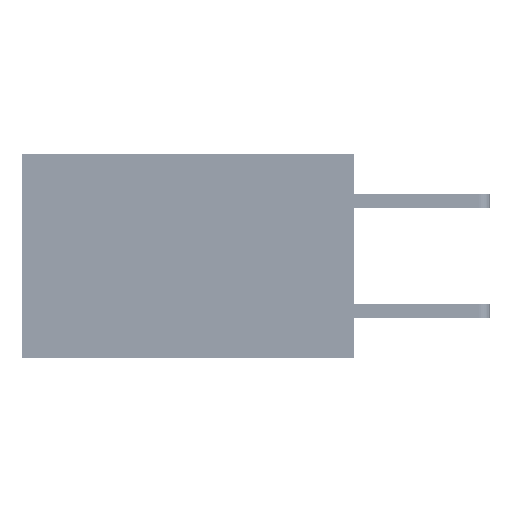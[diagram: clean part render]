
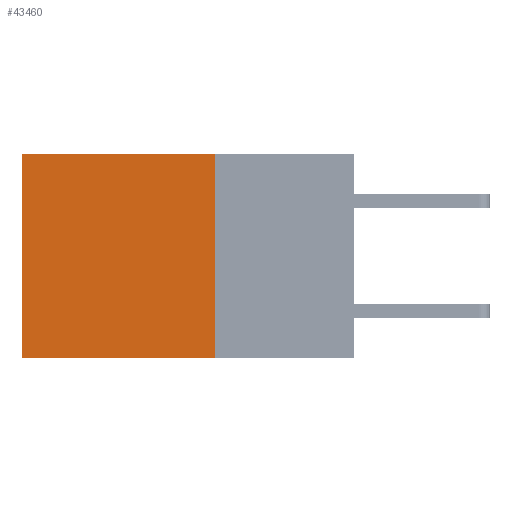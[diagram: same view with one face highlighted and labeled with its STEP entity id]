
A CAD part, left-side view. The second image highlights one B-rep face of the part: STEP entity #43460.
In plain terms, the highlighted planar face has unit normal (-1, 0, 0).
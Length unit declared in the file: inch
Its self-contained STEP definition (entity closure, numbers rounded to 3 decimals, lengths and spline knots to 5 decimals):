
#85 = CARTESIAN_POINT ( 'NONE',  ( 0.2875, 0.25, -0.37 ) ) ;
#1577 = EDGE_CURVE ( 'NONE', #25492, #35846, #40350, .T. ) ;
#1589 = ORIENTED_EDGE ( 'NONE', *, *, #36701, .F. ) ;
#4598 = ORIENTED_EDGE ( 'NONE', *, *, #1577, .T. ) ;
#4735 = CARTESIAN_POINT ( 'NONE',  ( 0.2875, 0.6, 0. ) ) ;
#4952 = VECTOR ( 'NONE', #6982, 39.37008 ) ;
#6982 = DIRECTION ( 'NONE',  ( 0., 1., 0. ) ) ;
#8713 = CARTESIAN_POINT ( 'NONE',  ( 0.2875, 0.25, 0. ) ) ;
#10041 = FACE_OUTER_BOUND ( 'NONE', #24986, .T. ) ;
#13218 = DIRECTION ( 'NONE',  ( 0., 0., -1. ) ) ;
#15176 = VERTEX_POINT ( 'NONE', #21913 ) ;
#15737 = DIRECTION ( 'NONE',  ( 0., 0., -1. ) ) ;
#17518 = CARTESIAN_POINT ( 'NONE',  ( 0.2875, 0.25, 0. ) ) ;
#18536 = EDGE_CURVE ( 'NONE', #28150, #25492, #32830, .T. ) ;
#19465 = ORIENTED_EDGE ( 'NONE', *, *, #37865, .F. ) ;
#20955 = DIRECTION ( 'NONE',  ( 0., 1., 0. ) ) ;
#21913 = CARTESIAN_POINT ( 'NONE',  ( 0.2875, 0.25, -0.37 ) ) ;
#23087 = VECTOR ( 'NONE', #20955, 39.37008 ) ;
#24986 = EDGE_LOOP ( 'NONE', ( #4598, #1589, #19465, #33748 ) ) ;
#25492 = VERTEX_POINT ( 'NONE', #4735 ) ;
#28150 = VERTEX_POINT ( 'NONE', #37398 ) ;
#30674 = VECTOR ( 'NONE', #13218, 39.37008 ) ;
#31085 = VECTOR ( 'NONE', #38498, 39.37008 ) ;
#32830 = LINE ( 'NONE', #17518, #4952 ) ;
#33113 = PLANE ( 'NONE',  #35309 ) ;
#33748 = ORIENTED_EDGE ( 'NONE', *, *, #18536, .T. ) ;
#35309 = AXIS2_PLACEMENT_3D ( 'NONE', #8713, #36637, #15737 ) ;
#35846 = VERTEX_POINT ( 'NONE', #44011 ) ;
#36637 = DIRECTION ( 'NONE',  ( 1., 0., 0. ) ) ;
#36701 = EDGE_CURVE ( 'NONE', #15176, #35846, #41699, .T. ) ;
#37398 = CARTESIAN_POINT ( 'NONE',  ( 0.2875, 0.25, 0. ) ) ;
#37626 = CARTESIAN_POINT ( 'NONE',  ( 0.2875, 0.25, 0. ) ) ;
#37865 = EDGE_CURVE ( 'NONE', #28150, #15176, #38895, .T. ) ;
#38109 = CARTESIAN_POINT ( 'NONE',  ( 0.2875, 0.6, 0. ) ) ;
#38498 = DIRECTION ( 'NONE',  ( 0., 0., -1. ) ) ;
#38895 = LINE ( 'NONE', #37626, #30674 ) ;
#40350 = LINE ( 'NONE', #38109, #31085 ) ;
#41699 = LINE ( 'NONE', #85, #23087 ) ;
#43460 = ADVANCED_FACE ( 'NONE', ( #10041 ), #33113, .F. ) ;
#44011 = CARTESIAN_POINT ( 'NONE',  ( 0.2875, 0.6, -0.37 ) ) ;
